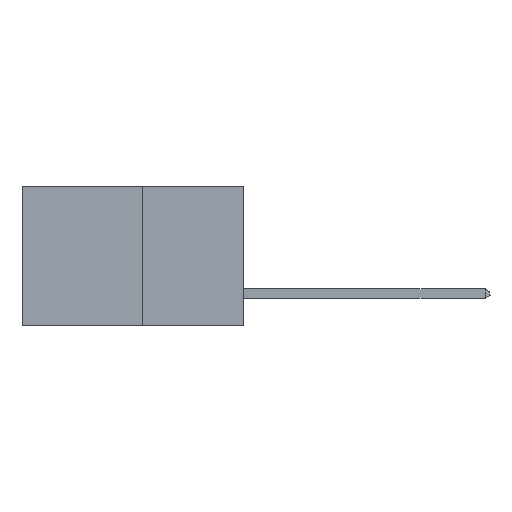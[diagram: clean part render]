
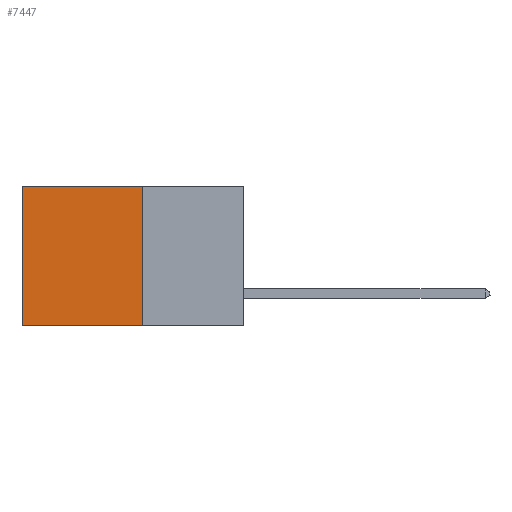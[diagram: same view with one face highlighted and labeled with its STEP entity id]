
A CAD part, left-side view. The second image highlights one B-rep face of the part: STEP entity #7447.
In plain terms, the highlighted planar face has unit normal (-1, 0, 0).
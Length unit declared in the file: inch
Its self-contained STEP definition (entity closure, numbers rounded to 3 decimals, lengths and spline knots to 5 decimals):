
#38 = CARTESIAN_POINT ( 'NONE',  ( 0.277, 0.27, 0. ) ) ;
#1145 = ORIENTED_EDGE ( 'NONE', *, *, #12619, .F. ) ;
#1213 = DIRECTION ( 'NONE',  ( 0., 0., -1. ) ) ;
#1299 = LINE ( 'NONE', #5074, #4425 ) ;
#2316 = EDGE_LOOP ( 'NONE', ( #10174, #7466, #1145, #8567 ) ) ;
#2389 = LINE ( 'NONE', #4760, #2757 ) ;
#2757 = VECTOR ( 'NONE', #1213, 39.37008 ) ;
#2848 = EDGE_CURVE ( 'NONE', #4912, #7491, #1299, .T. ) ;
#4425 = VECTOR ( 'NONE', #11986, 39.37008 ) ;
#4453 = VERTEX_POINT ( 'NONE', #38 ) ;
#4615 = CARTESIAN_POINT ( 'NONE',  ( 0.277, 0.59, 0. ) ) ;
#4760 = CARTESIAN_POINT ( 'NONE',  ( 0.277, 0.27, -0.37 ) ) ;
#4912 = VERTEX_POINT ( 'NONE', #4615 ) ;
#5074 = CARTESIAN_POINT ( 'NONE',  ( 0.277, 0.59, -0.37 ) ) ;
#5213 = CARTESIAN_POINT ( 'NONE',  ( 0.277, 0.59, -0.37 ) ) ;
#5221 = CARTESIAN_POINT ( 'NONE',  ( 0.277, 0.27, -0.37 ) ) ;
#6082 = VECTOR ( 'NONE', #14177, 39.37008 ) ;
#6104 = CARTESIAN_POINT ( 'NONE',  ( 0.277, 0.27, 0. ) ) ;
#6426 = DIRECTION ( 'NONE',  ( 0., 0., -1. ) ) ;
#6656 = FACE_OUTER_BOUND ( 'NONE', #2316, .T. ) ;
#7273 = EDGE_CURVE ( 'NONE', #4453, #4912, #11946, .T. ) ;
#7447 = ADVANCED_FACE ( 'NONE', ( #6656 ), #11093, .F. ) ;
#7466 = ORIENTED_EDGE ( 'NONE', *, *, #10573, .F. ) ;
#7491 = VERTEX_POINT ( 'NONE', #5213 ) ;
#8567 = ORIENTED_EDGE ( 'NONE', *, *, #7273, .T. ) ;
#8814 = VERTEX_POINT ( 'NONE', #14509 ) ;
#9052 = DIRECTION ( 'NONE',  ( 0., 1., 0. ) ) ;
#10174 = ORIENTED_EDGE ( 'NONE', *, *, #2848, .T. ) ;
#10573 = EDGE_CURVE ( 'NONE', #8814, #7491, #13971, .T. ) ;
#10618 = VECTOR ( 'NONE', #9052, 39.37008 ) ;
#10952 = AXIS2_PLACEMENT_3D ( 'NONE', #5221, #13363, #6426 ) ;
#11093 = PLANE ( 'NONE',  #10952 ) ;
#11373 = CARTESIAN_POINT ( 'NONE',  ( 0.277, 0.27, -0.37 ) ) ;
#11946 = LINE ( 'NONE', #6104, #6082 ) ;
#11986 = DIRECTION ( 'NONE',  ( 0., 0., -1. ) ) ;
#12619 = EDGE_CURVE ( 'NONE', #4453, #8814, #2389, .T. ) ;
#13363 = DIRECTION ( 'NONE',  ( 1., 0., 0. ) ) ;
#13971 = LINE ( 'NONE', #11373, #10618 ) ;
#14177 = DIRECTION ( 'NONE',  ( 0., 1., 0. ) ) ;
#14509 = CARTESIAN_POINT ( 'NONE',  ( 0.277, 0.27, -0.37 ) ) ;
